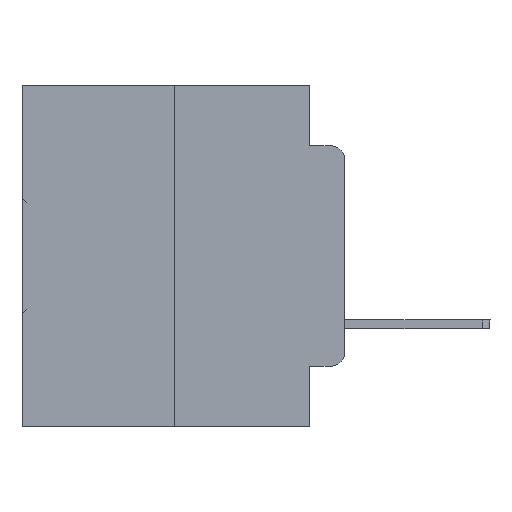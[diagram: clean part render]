
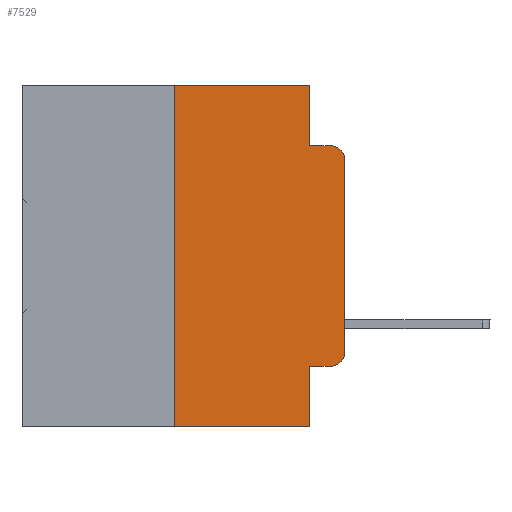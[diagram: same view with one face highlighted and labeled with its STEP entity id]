
A CAD part, left-side view. The second image highlights one B-rep face of the part: STEP entity #7529.
In plain terms, the highlighted planar face has unit normal (-1, 0, 0).
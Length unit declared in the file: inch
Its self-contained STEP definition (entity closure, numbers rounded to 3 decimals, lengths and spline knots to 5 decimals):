
#359 = DIRECTION ( 'NONE',  ( 0., -1., 0. ) ) ;
#424 = DIRECTION ( 'NONE',  ( 0., 0., 1. ) ) ;
#460 = CARTESIAN_POINT ( 'NONE',  ( 0., 0.473, -0.5 ) ) ;
#482 = CIRCLE ( 'NONE', #9150, 0.02 ) ;
#652 = CARTESIAN_POINT ( 'NONE',  ( 0., 0.051, 0. ) ) ;
#815 = LINE ( 'NONE', #652, #14197 ) ;
#874 = ORIENTED_EDGE ( 'NONE', *, *, #29799, .F. ) ;
#2143 = VERTEX_POINT ( 'NONE', #5143 ) ;
#2352 = LINE ( 'NONE', #14809, #16147 ) ;
#2829 = DIRECTION ( 'NONE',  ( 0., 0., 1. ) ) ;
#2953 = ORIENTED_EDGE ( 'NONE', *, *, #15093, .T. ) ;
#3240 = FACE_OUTER_BOUND ( 'NONE', #24703, .T. ) ;
#3312 = DIRECTION ( 'NONE',  ( 0., 0., -1. ) ) ;
#3809 = LINE ( 'NONE', #11004, #18224 ) ;
#4787 = DIRECTION ( 'NONE',  ( 0., -1., 0. ) ) ;
#4899 = VECTOR ( 'NONE', #359, 39.37008 ) ;
#5143 = CARTESIAN_POINT ( 'NONE',  ( 0., 0.25, 0. ) ) ;
#5260 = LINE ( 'NONE', #460, #18162 ) ;
#6153 = DIRECTION ( 'NONE',  ( -1., 0., 0. ) ) ;
#7119 = VERTEX_POINT ( 'NONE', #30428 ) ;
#7155 = LINE ( 'NONE', #17212, #28836 ) ;
#7529 = ADVANCED_FACE ( 'NONE', ( #3240 ), #22740, .F. ) ;
#8056 = CARTESIAN_POINT ( 'NONE',  ( 0., 0., -0.3915 ) ) ;
#8431 = ORIENTED_EDGE ( 'NONE', *, *, #19221, .T. ) ;
#8447 = VERTEX_POINT ( 'NONE', #8056 ) ;
#8619 = DIRECTION ( 'NONE',  ( 0., 0., -1. ) ) ;
#9059 = VECTOR ( 'NONE', #10430, 39.37008 ) ;
#9150 = AXIS2_PLACEMENT_3D ( 'NONE', #27760, #13526, #3312 ) ;
#9392 = CARTESIAN_POINT ( 'NONE',  ( 0., 0.051, -0.0885 ) ) ;
#10346 = EDGE_CURVE ( 'NONE', #20516, #7119, #815, .T. ) ;
#10430 = DIRECTION ( 'NONE',  ( 0., -1., 0. ) ) ;
#10769 = DIRECTION ( 'NONE',  ( 0., 0., -1. ) ) ;
#11004 = CARTESIAN_POINT ( 'NONE',  ( 0., 0.051, 0. ) ) ;
#11402 = VERTEX_POINT ( 'NONE', #21607 ) ;
#12067 = CARTESIAN_POINT ( 'NONE',  ( 0., 0., -0.1085 ) ) ;
#13433 = DIRECTION ( 'NONE',  ( 0., 0., -1. ) ) ;
#13526 = DIRECTION ( 'NONE',  ( -1., 0., 0. ) ) ;
#13677 = ORIENTED_EDGE ( 'NONE', *, *, #27506, .F. ) ;
#14088 = AXIS2_PLACEMENT_3D ( 'NONE', #22261, #29752, #10769 ) ;
#14197 = VECTOR ( 'NONE', #13433, 39.37008 ) ;
#14709 = EDGE_CURVE ( 'NONE', #17365, #30257, #5260, .T. ) ;
#14809 = CARTESIAN_POINT ( 'NONE',  ( 0., 0., 0. ) ) ;
#15093 = EDGE_CURVE ( 'NONE', #8447, #16847, #2352, .T. ) ;
#15221 = LINE ( 'NONE', #17456, #9059 ) ;
#15258 = ORIENTED_EDGE ( 'NONE', *, *, #17381, .F. ) ;
#15775 = AXIS2_PLACEMENT_3D ( 'NONE', #17981, #6153, #25611 ) ;
#16147 = VECTOR ( 'NONE', #424, 39.37008 ) ;
#16298 = CARTESIAN_POINT ( 'NONE',  ( 0., 0.051, 0. ) ) ;
#16847 = VERTEX_POINT ( 'NONE', #12067 ) ;
#17206 = LINE ( 'NONE', #9392, #26382 ) ;
#17212 = CARTESIAN_POINT ( 'NONE',  ( 0., 0.25, 0. ) ) ;
#17365 = VERTEX_POINT ( 'NONE', #27345 ) ;
#17381 = EDGE_CURVE ( 'NONE', #11402, #30257, #3809, .T. ) ;
#17456 = CARTESIAN_POINT ( 'NONE',  ( 0., 0.051, -0.4115 ) ) ;
#17981 = CARTESIAN_POINT ( 'NONE',  ( 0., 0.02, -0.1085 ) ) ;
#18074 = CARTESIAN_POINT ( 'NONE',  ( 0., 0.02, -0.4115 ) ) ;
#18162 = VECTOR ( 'NONE', #4787, 39.37008 ) ;
#18224 = VECTOR ( 'NONE', #8619, 39.37008 ) ;
#18293 = ORIENTED_EDGE ( 'NONE', *, *, #10346, .F. ) ;
#18763 = ORIENTED_EDGE ( 'NONE', *, *, #14709, .T. ) ;
#19128 = DIRECTION ( 'NONE',  ( 0., -1., 0. ) ) ;
#19221 = EDGE_CURVE ( 'NONE', #27429, #8447, #482, .T. ) ;
#19550 = EDGE_CURVE ( 'NONE', #16847, #30196, #29552, .T. ) ;
#20203 = ORIENTED_EDGE ( 'NONE', *, *, #19550, .T. ) ;
#20516 = VERTEX_POINT ( 'NONE', #16298 ) ;
#21607 = CARTESIAN_POINT ( 'NONE',  ( 0., 0.051, -0.4115 ) ) ;
#22148 = ORIENTED_EDGE ( 'NONE', *, *, #30996, .F. ) ;
#22261 = CARTESIAN_POINT ( 'NONE',  ( 0., 0.473, 0. ) ) ;
#22740 = PLANE ( 'NONE',  #14088 ) ;
#24703 = EDGE_LOOP ( 'NONE', ( #2953, #20203, #22148, #18293, #874, #13677, #18763, #15258, #25821, #8431 ) ) ;
#25611 = DIRECTION ( 'NONE',  ( 0., 0., -1. ) ) ;
#25821 = ORIENTED_EDGE ( 'NONE', *, *, #29773, .T. ) ;
#26382 = VECTOR ( 'NONE', #19128, 39.37008 ) ;
#27207 = CARTESIAN_POINT ( 'NONE',  ( 0., 0.02, -0.0885 ) ) ;
#27345 = CARTESIAN_POINT ( 'NONE',  ( 0., 0.25, -0.5 ) ) ;
#27429 = VERTEX_POINT ( 'NONE', #18074 ) ;
#27506 = EDGE_CURVE ( 'NONE', #17365, #2143, #7155, .T. ) ;
#27760 = CARTESIAN_POINT ( 'NONE',  ( 0., 0.02, -0.3915 ) ) ;
#28836 = VECTOR ( 'NONE', #2829, 39.37008 ) ;
#29552 = CIRCLE ( 'NONE', #15775, 0.02 ) ;
#29586 = CARTESIAN_POINT ( 'NONE',  ( 0., 0.473, 0. ) ) ;
#29604 = CARTESIAN_POINT ( 'NONE',  ( 0., 0.051, -0.5 ) ) ;
#29752 = DIRECTION ( 'NONE',  ( 1., 0., 0. ) ) ;
#29773 = EDGE_CURVE ( 'NONE', #11402, #27429, #15221, .T. ) ;
#29799 = EDGE_CURVE ( 'NONE', #2143, #20516, #30056, .T. ) ;
#30056 = LINE ( 'NONE', #29586, #4899 ) ;
#30196 = VERTEX_POINT ( 'NONE', #27207 ) ;
#30257 = VERTEX_POINT ( 'NONE', #29604 ) ;
#30428 = CARTESIAN_POINT ( 'NONE',  ( 0., 0.051, -0.0885 ) ) ;
#30996 = EDGE_CURVE ( 'NONE', #7119, #30196, #17206, .T. ) ;
